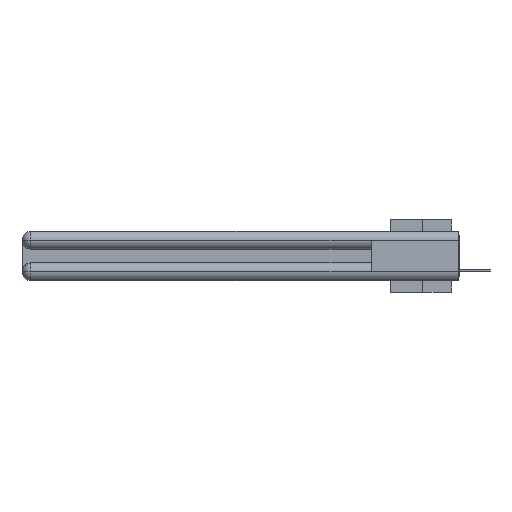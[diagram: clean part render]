
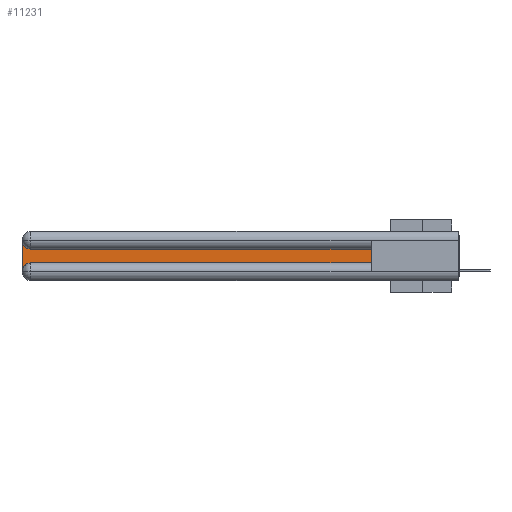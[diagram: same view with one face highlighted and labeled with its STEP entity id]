
A CAD part, left-side view. The second image highlights one B-rep face of the part: STEP entity #11231.
In plain terms, the highlighted planar face has unit normal (-1, 0, 0).
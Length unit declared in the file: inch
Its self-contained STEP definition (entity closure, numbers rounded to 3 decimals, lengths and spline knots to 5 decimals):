
#117 = EDGE_CURVE ( 'NONE', #15181, #18947, #18716, .T. ) ;
#2346 = VECTOR ( 'NONE', #25107, 39.37008 ) ;
#2377 = AXIS2_PLACEMENT_3D ( 'NONE', #17109, #31450, #6783 ) ;
#3099 = VERTEX_POINT ( 'NONE', #31194 ) ;
#3134 = CARTESIAN_POINT ( 'NONE',  ( 0.075, 3., -0.2175 ) ) ;
#4441 = CARTESIAN_POINT ( 'NONE',  ( 0.075, 3., -0.0625 ) ) ;
#4705 = CARTESIAN_POINT ( 'NONE',  ( 0.075, 2.94, -0.1225 ) ) ;
#5012 = DIRECTION ( 'NONE',  ( 0., 1., 0. ) ) ;
#5015 = DIRECTION ( 'NONE',  ( 0., 0., 1. ) ) ;
#5176 = LINE ( 'NONE', #30942, #23843 ) ;
#5542 = DIRECTION ( 'NONE',  ( 1., 0., 0. ) ) ;
#6680 = ORIENTED_EDGE ( 'NONE', *, *, #17891, .T. ) ;
#6754 = EDGE_CURVE ( 'NONE', #31811, #24601, #22570, .T. ) ;
#6783 = DIRECTION ( 'NONE',  ( 0., 0., -1. ) ) ;
#7055 = CIRCLE ( 'NONE', #11337, 0.06 ) ;
#7837 = CARTESIAN_POINT ( 'NONE',  ( 0.075, 2.94, -0.2775 ) ) ;
#7964 = CARTESIAN_POINT ( 'NONE',  ( 0.075, 3., -0.1225 ) ) ;
#8152 = DIRECTION ( 'NONE',  ( 1., 0., 0. ) ) ;
#8353 = CARTESIAN_POINT ( 'NONE',  ( 0.075, 0.6, -0.1225 ) ) ;
#8682 = ORIENTED_EDGE ( 'NONE', *, *, #6754, .T. ) ;
#9385 = EDGE_CURVE ( 'NONE', #24601, #15181, #14164, .T. ) ;
#10560 = DIRECTION ( 'NONE',  ( 0., 0., -1. ) ) ;
#11231 = ADVANCED_FACE ( 'NONE', ( #21435 ), #12827, .F. ) ;
#11337 = AXIS2_PLACEMENT_3D ( 'NONE', #7837, #8152, #27747 ) ;
#11370 = CARTESIAN_POINT ( 'NONE',  ( 0.075, 0.6, -0.1225 ) ) ;
#12827 = PLANE ( 'NONE',  #21093 ) ;
#14164 = LINE ( 'NONE', #8353, #16499 ) ;
#15181 = VERTEX_POINT ( 'NONE', #4705 ) ;
#15819 = ORIENTED_EDGE ( 'NONE', *, *, #117, .T. ) ;
#16040 = VERTEX_POINT ( 'NONE', #26542 ) ;
#16410 = ORIENTED_EDGE ( 'NONE', *, *, #9385, .T. ) ;
#16499 = VECTOR ( 'NONE', #5012, 39.37008 ) ;
#17109 = CARTESIAN_POINT ( 'NONE',  ( 0.075, 2.94, -0.0625 ) ) ;
#17891 = EDGE_CURVE ( 'NONE', #16040, #3099, #7055, .T. ) ;
#18716 = CIRCLE ( 'NONE', #2377, 0.06 ) ;
#18947 = VERTEX_POINT ( 'NONE', #4441 ) ;
#19086 = ORIENTED_EDGE ( 'NONE', *, *, #22567, .T. ) ;
#21093 = AXIS2_PLACEMENT_3D ( 'NONE', #7964, #5542, #10560 ) ;
#21248 = EDGE_LOOP ( 'NONE', ( #16410, #15819, #19086, #6680, #31681, #8682 ) ) ;
#21345 = LINE ( 'NONE', #3134, #2346 ) ;
#21435 = FACE_OUTER_BOUND ( 'NONE', #21248, .T. ) ;
#21819 = CARTESIAN_POINT ( 'NONE',  ( 0.075, 0.6, -0.2175 ) ) ;
#22567 = EDGE_CURVE ( 'NONE', #18947, #16040, #21345, .T. ) ;
#22570 = LINE ( 'NONE', #31760, #26416 ) ;
#23415 = DIRECTION ( 'NONE',  ( 0., -1., 0. ) ) ;
#23843 = VECTOR ( 'NONE', #23415, 39.37008 ) ;
#24601 = VERTEX_POINT ( 'NONE', #11370 ) ;
#25107 = DIRECTION ( 'NONE',  ( 0., 0., -1. ) ) ;
#25288 = EDGE_CURVE ( 'NONE', #3099, #31811, #5176, .T. ) ;
#26416 = VECTOR ( 'NONE', #5015, 39.37008 ) ;
#26542 = CARTESIAN_POINT ( 'NONE',  ( 0.075, 3., -0.2775 ) ) ;
#27747 = DIRECTION ( 'NONE',  ( 0., 0., -1. ) ) ;
#30942 = CARTESIAN_POINT ( 'NONE',  ( 0.075, 0.6, -0.2175 ) ) ;
#31194 = CARTESIAN_POINT ( 'NONE',  ( 0.075, 2.94, -0.2175 ) ) ;
#31450 = DIRECTION ( 'NONE',  ( 1., 0., 0. ) ) ;
#31681 = ORIENTED_EDGE ( 'NONE', *, *, #25288, .T. ) ;
#31760 = CARTESIAN_POINT ( 'NONE',  ( 0.075, 0.6, -0.2175 ) ) ;
#31811 = VERTEX_POINT ( 'NONE', #21819 ) ;
